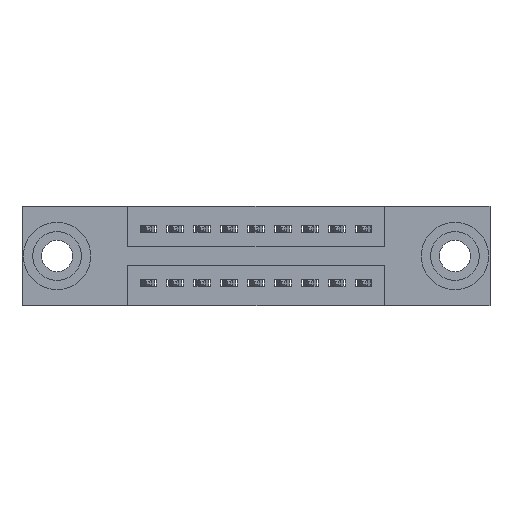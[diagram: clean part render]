
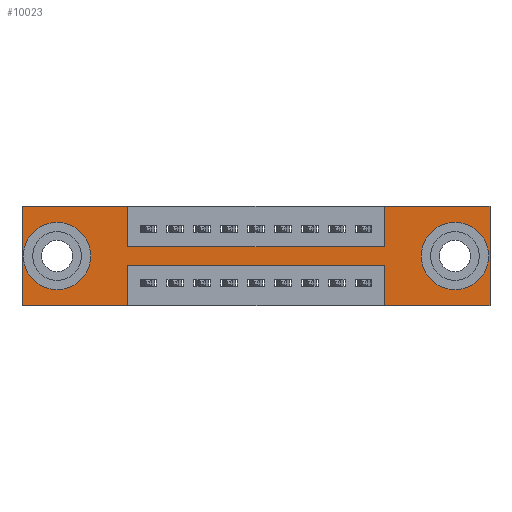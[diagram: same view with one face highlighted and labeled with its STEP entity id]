
A CAD part, front view. The second image highlights one B-rep face of the part: STEP entity #10023.
In plain terms, the highlighted planar face has unit normal (0, -1, 0).
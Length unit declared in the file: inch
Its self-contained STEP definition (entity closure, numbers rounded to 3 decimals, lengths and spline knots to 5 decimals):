
#151 = CARTESIAN_POINT ( 'NONE',  ( 0.3925, 0., -0.37 ) ) ;
#154 = VERTEX_POINT ( 'NONE', #4886 ) ;
#160 = CARTESIAN_POINT ( 'NONE',  ( 1.605, 0., -0.263 ) ) ;
#170 = EDGE_CURVE ( 'NONE', #6784, #4953, #1347, .T. ) ;
#319 = LINE ( 'NONE', #811, #11345 ) ;
#386 = FACE_OUTER_BOUND ( 'NONE', #3245, .T. ) ;
#437 = VECTOR ( 'NONE', #3868, 39.37008 ) ;
#456 = CARTESIAN_POINT ( 'NONE',  ( 1.3425, 0., 0. ) ) ;
#752 = VERTEX_POINT ( 'NONE', #5394 ) ;
#811 = CARTESIAN_POINT ( 'NONE',  ( 0., 0., -0.37 ) ) ;
#834 = ORIENTED_EDGE ( 'NONE', *, *, #4954, .F. ) ;
#903 = EDGE_CURVE ( 'NONE', #10817, #752, #3980, .T. ) ;
#1034 = CARTESIAN_POINT ( 'NONE',  ( 0.3925, 0., -0.15 ) ) ;
#1202 = CARTESIAN_POINT ( 'NONE',  ( 1.3425, 0., -0.37 ) ) ;
#1240 = CARTESIAN_POINT ( 'NONE',  ( 1.605, 0., -0.185 ) ) ;
#1347 = LINE ( 'NONE', #2416, #4897 ) ;
#1375 = EDGE_CURVE ( 'NONE', #5132, #4968, #7400, .T. ) ;
#1568 = VERTEX_POINT ( 'NONE', #7639 ) ;
#1628 = CARTESIAN_POINT ( 'NONE',  ( 0.3925, 0., 0. ) ) ;
#1686 = DIRECTION ( 'NONE',  ( 0., 0., -1. ) ) ;
#1788 = LINE ( 'NONE', #1034, #3654 ) ;
#1829 = ORIENTED_EDGE ( 'NONE', *, *, #3105, .F. ) ;
#2072 = AXIS2_PLACEMENT_3D ( 'NONE', #11747, #10931, #3229 ) ;
#2131 = CARTESIAN_POINT ( 'NONE',  ( 0., 0., 0. ) ) ;
#2239 = VECTOR ( 'NONE', #7385, 39.37008 ) ;
#2328 = EDGE_CURVE ( 'NONE', #4968, #5132, #2766, .T. ) ;
#2393 = DIRECTION ( 'NONE',  ( 1., 0., 0. ) ) ;
#2416 = CARTESIAN_POINT ( 'NONE',  ( 0., 0., 0. ) ) ;
#2459 = CARTESIAN_POINT ( 'NONE',  ( 0.3925, 0., 0. ) ) ;
#2525 = LINE ( 'NONE', #2131, #2239 ) ;
#2605 = AXIS2_PLACEMENT_3D ( 'NONE', #8342, #4584, #11227 ) ;
#2644 = ORIENTED_EDGE ( 'NONE', *, *, #11247, .F. ) ;
#2652 = ORIENTED_EDGE ( 'NONE', *, *, #7655, .F. ) ;
#2766 = CIRCLE ( 'NONE', #2072, 0.078 ) ;
#2994 = DIRECTION ( 'NONE',  ( 0., 0., -1. ) ) ;
#3059 = LINE ( 'NONE', #6285, #9119 ) ;
#3105 = EDGE_CURVE ( 'NONE', #12099, #154, #5547, .T. ) ;
#3229 = DIRECTION ( 'NONE',  ( 0., 0., 1. ) ) ;
#3245 = EDGE_LOOP ( 'NONE', ( #10267, #11350, #2652, #3283, #834, #5128, #1829, #7027, #2644, #4252, #12118, #10148 ) ) ;
#3247 = ORIENTED_EDGE ( 'NONE', *, *, #903, .T. ) ;
#3283 = ORIENTED_EDGE ( 'NONE', *, *, #6436, .F. ) ;
#3418 = DIRECTION ( 'NONE',  ( 0., 0., -1. ) ) ;
#3654 = VECTOR ( 'NONE', #2393, 39.37008 ) ;
#3868 = DIRECTION ( 'NONE',  ( 0., 0., 1. ) ) ;
#3980 = CIRCLE ( 'NONE', #4500, 0.078 ) ;
#4109 = PLANE ( 'NONE',  #8846 ) ;
#4252 = ORIENTED_EDGE ( 'NONE', *, *, #170, .F. ) ;
#4309 = ORIENTED_EDGE ( 'NONE', *, *, #1375, .T. ) ;
#4404 = CARTESIAN_POINT ( 'NONE',  ( 1.605, 0., -0.185 ) ) ;
#4477 = VERTEX_POINT ( 'NONE', #10354 ) ;
#4500 = AXIS2_PLACEMENT_3D ( 'NONE', #1240, #5906, #7848 ) ;
#4584 = DIRECTION ( 'NONE',  ( 0., 1., 0. ) ) ;
#4732 = EDGE_LOOP ( 'NONE', ( #5528, #4309 ) ) ;
#4863 = LINE ( 'NONE', #7071, #11318 ) ;
#4886 = CARTESIAN_POINT ( 'NONE',  ( 1.3425, 0., 0. ) ) ;
#4897 = VECTOR ( 'NONE', #10721, 39.37008 ) ;
#4953 = VERTEX_POINT ( 'NONE', #2459 ) ;
#4954 = EDGE_CURVE ( 'NONE', #7672, #6056, #7593, .T. ) ;
#4968 = VERTEX_POINT ( 'NONE', #9198 ) ;
#5128 = ORIENTED_EDGE ( 'NONE', *, *, #10143, .F. ) ;
#5132 = VERTEX_POINT ( 'NONE', #5226 ) ;
#5226 = CARTESIAN_POINT ( 'NONE',  ( 0.13, 0., -0.263 ) ) ;
#5394 = CARTESIAN_POINT ( 'NONE',  ( 1.605, 0., -0.107 ) ) ;
#5422 = DIRECTION ( 'NONE',  ( 0., 1., 0. ) ) ;
#5528 = ORIENTED_EDGE ( 'NONE', *, *, #2328, .T. ) ;
#5547 = LINE ( 'NONE', #456, #10277 ) ;
#5906 = DIRECTION ( 'NONE',  ( 0., 1., 0. ) ) ;
#5959 = CARTESIAN_POINT ( 'NONE',  ( 1.3425, 0., -0.15 ) ) ;
#6056 = VERTEX_POINT ( 'NONE', #11592 ) ;
#6177 = DIRECTION ( 'NONE',  ( 0., 0., -1. ) ) ;
#6285 = CARTESIAN_POINT ( 'NONE',  ( 0.3925, 0., -0.22 ) ) ;
#6325 = DIRECTION ( 'NONE',  ( 0., 0., -1. ) ) ;
#6411 = DIRECTION ( 'NONE',  ( -1., 0., 0. ) ) ;
#6436 = EDGE_CURVE ( 'NONE', #6056, #7531, #319, .T. ) ;
#6589 = CIRCLE ( 'NONE', #11805, 0.078 ) ;
#6711 = VECTOR ( 'NONE', #7850, 39.37008 ) ;
#6784 = VERTEX_POINT ( 'NONE', #8603 ) ;
#7027 = ORIENTED_EDGE ( 'NONE', *, *, #7951, .F. ) ;
#7071 = CARTESIAN_POINT ( 'NONE',  ( 0., 0., -0.37 ) ) ;
#7265 = CARTESIAN_POINT ( 'NONE',  ( 1.3425, 0., -0.37 ) ) ;
#7306 = EDGE_CURVE ( 'NONE', #1568, #6784, #2525, .T. ) ;
#7354 = CARTESIAN_POINT ( 'NONE',  ( 0.3925, 0., -0.37 ) ) ;
#7375 = CARTESIAN_POINT ( 'NONE',  ( 1.735, 0., 0. ) ) ;
#7385 = DIRECTION ( 'NONE',  ( 0., 0., 1. ) ) ;
#7400 = CIRCLE ( 'NONE', #2605, 0.078 ) ;
#7531 = VERTEX_POINT ( 'NONE', #7265 ) ;
#7593 = LINE ( 'NONE', #7375, #7899 ) ;
#7639 = CARTESIAN_POINT ( 'NONE',  ( 0., 0., -0.37 ) ) ;
#7655 = EDGE_CURVE ( 'NONE', #7531, #11042, #7824, .T. ) ;
#7672 = VERTEX_POINT ( 'NONE', #8725 ) ;
#7721 = EDGE_CURVE ( 'NONE', #10573, #1568, #4863, .T. ) ;
#7807 = EDGE_LOOP ( 'NONE', ( #8918, #3247 ) ) ;
#7824 = LINE ( 'NONE', #1202, #437 ) ;
#7848 = DIRECTION ( 'NONE',  ( 0., 0., -1. ) ) ;
#7850 = DIRECTION ( 'NONE',  ( 1., 0., 0. ) ) ;
#7899 = VECTOR ( 'NONE', #6325, 39.37008 ) ;
#7951 = EDGE_CURVE ( 'NONE', #4477, #12099, #1788, .T. ) ;
#8016 = CARTESIAN_POINT ( 'NONE',  ( 0., 0., -0.37 ) ) ;
#8190 = VERTEX_POINT ( 'NONE', #12127 ) ;
#8342 = CARTESIAN_POINT ( 'NONE',  ( 0.13, 0., -0.185 ) ) ;
#8390 = LINE ( 'NONE', #151, #10281 ) ;
#8413 = EDGE_CURVE ( 'NONE', #11042, #8190, #3059, .T. ) ;
#8513 = FACE_BOUND ( 'NONE', #7807, .T. ) ;
#8603 = CARTESIAN_POINT ( 'NONE',  ( 0., 0., 0. ) ) ;
#8725 = CARTESIAN_POINT ( 'NONE',  ( 1.735, 0., 0. ) ) ;
#8846 = AXIS2_PLACEMENT_3D ( 'NONE', #8016, #10868, #6177 ) ;
#8918 = ORIENTED_EDGE ( 'NONE', *, *, #12023, .T. ) ;
#9119 = VECTOR ( 'NONE', #6411, 39.37008 ) ;
#9198 = CARTESIAN_POINT ( 'NONE',  ( 0.13, 0., -0.107 ) ) ;
#9221 = FACE_BOUND ( 'NONE', #4732, .T. ) ;
#9625 = CARTESIAN_POINT ( 'NONE',  ( 0., 0., 0. ) ) ;
#9792 = DIRECTION ( 'NONE',  ( -1., 0., 0. ) ) ;
#9822 = VECTOR ( 'NONE', #3418, 39.37008 ) ;
#9870 = CARTESIAN_POINT ( 'NONE',  ( 1.3425, 0., -0.22 ) ) ;
#10023 = ADVANCED_FACE ( 'NONE', ( #8513, #9221, #386 ), #4109, .T. ) ;
#10143 = EDGE_CURVE ( 'NONE', #154, #7672, #10702, .T. ) ;
#10148 = ORIENTED_EDGE ( 'NONE', *, *, #7721, .F. ) ;
#10245 = DIRECTION ( 'NONE',  ( -1., 0., 0. ) ) ;
#10267 = ORIENTED_EDGE ( 'NONE', *, *, #11305, .F. ) ;
#10277 = VECTOR ( 'NONE', #11765, 39.37008 ) ;
#10281 = VECTOR ( 'NONE', #2994, 39.37008 ) ;
#10354 = CARTESIAN_POINT ( 'NONE',  ( 0.3925, 0., -0.15 ) ) ;
#10573 = VERTEX_POINT ( 'NONE', #7354 ) ;
#10702 = LINE ( 'NONE', #9625, #6711 ) ;
#10721 = DIRECTION ( 'NONE',  ( 1., 0., 0. ) ) ;
#10817 = VERTEX_POINT ( 'NONE', #160 ) ;
#10868 = DIRECTION ( 'NONE',  ( 0., -1., 0. ) ) ;
#10931 = DIRECTION ( 'NONE',  ( 0., 1., 0. ) ) ;
#11042 = VERTEX_POINT ( 'NONE', #9870 ) ;
#11227 = DIRECTION ( 'NONE',  ( 0., 0., 1. ) ) ;
#11247 = EDGE_CURVE ( 'NONE', #4953, #4477, #11737, .T. ) ;
#11305 = EDGE_CURVE ( 'NONE', #8190, #10573, #8390, .T. ) ;
#11318 = VECTOR ( 'NONE', #9792, 39.37008 ) ;
#11345 = VECTOR ( 'NONE', #10245, 39.37008 ) ;
#11350 = ORIENTED_EDGE ( 'NONE', *, *, #8413, .F. ) ;
#11592 = CARTESIAN_POINT ( 'NONE',  ( 1.735, 0., -0.37 ) ) ;
#11737 = LINE ( 'NONE', #1628, #9822 ) ;
#11747 = CARTESIAN_POINT ( 'NONE',  ( 0.13, 0., -0.185 ) ) ;
#11765 = DIRECTION ( 'NONE',  ( 0., 0., 1. ) ) ;
#11805 = AXIS2_PLACEMENT_3D ( 'NONE', #4404, #5422, #1686 ) ;
#12023 = EDGE_CURVE ( 'NONE', #752, #10817, #6589, .T. ) ;
#12099 = VERTEX_POINT ( 'NONE', #5959 ) ;
#12118 = ORIENTED_EDGE ( 'NONE', *, *, #7306, .F. ) ;
#12127 = CARTESIAN_POINT ( 'NONE',  ( 0.3925, 0., -0.22 ) ) ;
